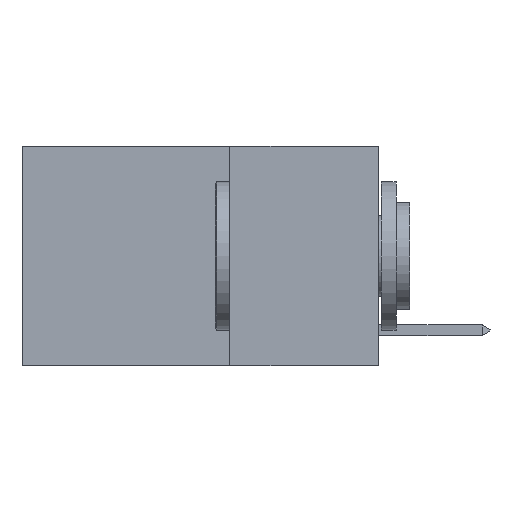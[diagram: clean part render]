
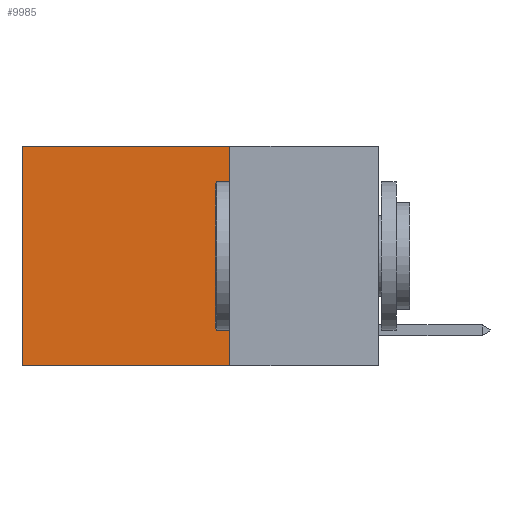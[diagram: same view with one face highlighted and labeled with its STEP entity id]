
A CAD part, left-side view. The second image highlights one B-rep face of the part: STEP entity #9985.
In plain terms, the highlighted planar face has unit normal (-1, 0, 0).
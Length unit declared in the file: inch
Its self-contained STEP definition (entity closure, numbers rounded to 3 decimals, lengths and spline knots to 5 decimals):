
#216 = EDGE_CURVE ( 'NONE', #1668, #7227, #4420, .T. ) ;
#331 = VECTOR ( 'NONE', #2331, 39.37008 ) ;
#871 = EDGE_CURVE ( 'NONE', #1668, #4630, #6881, .T. ) ;
#1668 = VERTEX_POINT ( 'NONE', #2349 ) ;
#1990 = VECTOR ( 'NONE', #5738, 39.37008 ) ;
#2004 = CARTESIAN_POINT ( 'NONE',  ( 0.2625, 0.25, 0. ) ) ;
#2114 = VECTOR ( 'NONE', #9644, 39.37008 ) ;
#2247 = EDGE_CURVE ( 'NONE', #4630, #6366, #9847, .T. ) ;
#2331 = DIRECTION ( 'NONE',  ( 0., 1., 0. ) ) ;
#2349 = CARTESIAN_POINT ( 'NONE',  ( 0.2625, 0.25, 0. ) ) ;
#2522 = VECTOR ( 'NONE', #8608, 39.37008 ) ;
#2996 = DIRECTION ( 'NONE',  ( 0., 0., -1. ) ) ;
#3114 = ORIENTED_EDGE ( 'NONE', *, *, #216, .F. ) ;
#4420 = LINE ( 'NONE', #7761, #1990 ) ;
#4630 = VERTEX_POINT ( 'NONE', #10672 ) ;
#5251 = CARTESIAN_POINT ( 'NONE',  ( 0.2625, 0.25, 0. ) ) ;
#5708 = EDGE_CURVE ( 'NONE', #7227, #6366, #9940, .T. ) ;
#5738 = DIRECTION ( 'NONE',  ( 0., 0., -1. ) ) ;
#5954 = CARTESIAN_POINT ( 'NONE',  ( 0.2625, 0.6, 0. ) ) ;
#6366 = VERTEX_POINT ( 'NONE', #8328 ) ;
#6881 = LINE ( 'NONE', #5251, #2114 ) ;
#7198 = EDGE_LOOP ( 'NONE', ( #7495, #9822, #3114, #10091 ) ) ;
#7227 = VERTEX_POINT ( 'NONE', #10786 ) ;
#7373 = PLANE ( 'NONE',  #11384 ) ;
#7495 = ORIENTED_EDGE ( 'NONE', *, *, #2247, .T. ) ;
#7761 = CARTESIAN_POINT ( 'NONE',  ( 0.2625, 0.25, 0. ) ) ;
#8241 = DIRECTION ( 'NONE',  ( 1., 0., 0. ) ) ;
#8328 = CARTESIAN_POINT ( 'NONE',  ( 0.2625, 0.6, -0.37 ) ) ;
#8608 = DIRECTION ( 'NONE',  ( 0., 0., -1. ) ) ;
#9644 = DIRECTION ( 'NONE',  ( 0., 1., 0. ) ) ;
#9822 = ORIENTED_EDGE ( 'NONE', *, *, #5708, .F. ) ;
#9847 = LINE ( 'NONE', #5954, #2522 ) ;
#9940 = LINE ( 'NONE', #10277, #331 ) ;
#9985 = ADVANCED_FACE ( 'NONE', ( #11755 ), #7373, .F. ) ;
#10091 = ORIENTED_EDGE ( 'NONE', *, *, #871, .T. ) ;
#10277 = CARTESIAN_POINT ( 'NONE',  ( 0.2625, 0.25, -0.37 ) ) ;
#10672 = CARTESIAN_POINT ( 'NONE',  ( 0.2625, 0.6, 0. ) ) ;
#10786 = CARTESIAN_POINT ( 'NONE',  ( 0.2625, 0.25, -0.37 ) ) ;
#11384 = AXIS2_PLACEMENT_3D ( 'NONE', #2004, #8241, #2996 ) ;
#11755 = FACE_OUTER_BOUND ( 'NONE', #7198, .T. ) ;
